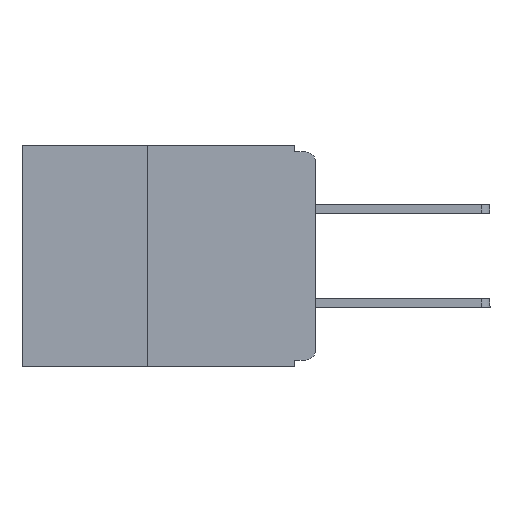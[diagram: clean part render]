
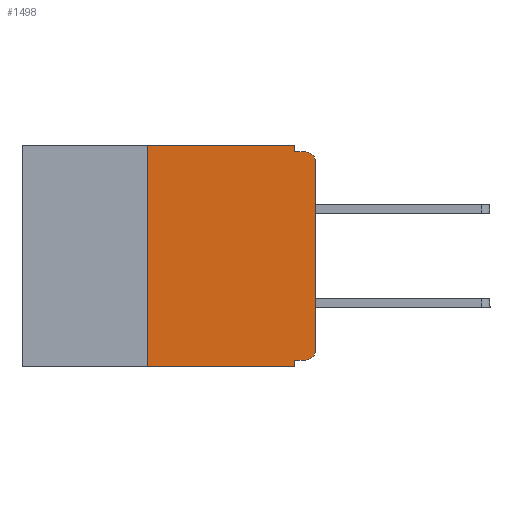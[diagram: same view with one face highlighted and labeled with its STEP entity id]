
A CAD part, left-side view. The second image highlights one B-rep face of the part: STEP entity #1498.
In plain terms, the highlighted planar face has unit normal (-1, 0, 0).
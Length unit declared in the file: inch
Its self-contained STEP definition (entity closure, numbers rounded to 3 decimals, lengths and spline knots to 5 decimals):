
#37 = EDGE_CURVE ( 'NONE', #2115, #16838, #28024, .T. ) ;
#264 = ORIENTED_EDGE ( 'NONE', *, *, #444, .F. ) ;
#444 = EDGE_CURVE ( 'NONE', #13419, #17743, #670, .T. ) ;
#670 = LINE ( 'NONE', #13961, #29350 ) ;
#885 = EDGE_CURVE ( 'NONE', #16838, #13419, #19014, .T. ) ;
#1094 = VECTOR ( 'NONE', #3043, 39.37008 ) ;
#1378 = DIRECTION ( 'NONE',  ( 0., -1., 0. ) ) ;
#1498 = ADVANCED_FACE ( 'NONE', ( #3923 ), #4084, .F. ) ;
#1636 = DIRECTION ( 'NONE',  ( -1., 0., 0. ) ) ;
#2097 = ORIENTED_EDGE ( 'NONE', *, *, #2987, .T. ) ;
#2115 = VERTEX_POINT ( 'NONE', #3869 ) ;
#2159 = CARTESIAN_POINT ( 'NONE',  ( 0., 0.437, -0.33 ) ) ;
#2605 = DIRECTION ( 'NONE',  ( 0., 0., -1. ) ) ;
#2610 = DIRECTION ( 'NONE',  ( 1., 0., 0. ) ) ;
#2978 = VERTEX_POINT ( 'NONE', #29318 ) ;
#2987 = EDGE_CURVE ( 'NONE', #21631, #26021, #19254, .T. ) ;
#3004 = VERTEX_POINT ( 'NONE', #22852 ) ;
#3043 = DIRECTION ( 'NONE',  ( 0., 0., -1. ) ) ;
#3101 = CARTESIAN_POINT ( 'NONE',  ( 0., 0.437, 0. ) ) ;
#3481 = CARTESIAN_POINT ( 'NONE',  ( 0., 0., -0.32 ) ) ;
#3617 = ORIENTED_EDGE ( 'NONE', *, *, #19073, .F. ) ;
#3869 = CARTESIAN_POINT ( 'NONE',  ( 0., 0.25, -0.33 ) ) ;
#3923 = FACE_OUTER_BOUND ( 'NONE', #14783, .T. ) ;
#3926 = VERTEX_POINT ( 'NONE', #7951 ) ;
#4084 = PLANE ( 'NONE',  #15643 ) ;
#4756 = LINE ( 'NONE', #3481, #16210 ) ;
#6631 = EDGE_CURVE ( 'NONE', #2115, #3926, #27111, .T. ) ;
#7951 = CARTESIAN_POINT ( 'NONE',  ( 0., 0.031, -0.33 ) ) ;
#8381 = AXIS2_PLACEMENT_3D ( 'NONE', #15422, #1636, #17712 ) ;
#8557 = CARTESIAN_POINT ( 'NONE',  ( 0., 0.015, -0.01 ) ) ;
#9186 = DIRECTION ( 'NONE',  ( 0., -1., 0. ) ) ;
#9751 = CARTESIAN_POINT ( 'NONE',  ( 0., 0.031, -0.01 ) ) ;
#9944 = DIRECTION ( 'NONE',  ( 0., 0., 1. ) ) ;
#10419 = CARTESIAN_POINT ( 'NONE',  ( 0., 0., -0.025 ) ) ;
#10887 = VECTOR ( 'NONE', #1378, 39.37008 ) ;
#11634 = DIRECTION ( 'NONE',  ( -1., 0., 0. ) ) ;
#11782 = CIRCLE ( 'NONE', #8381, 0.015 ) ;
#11783 = CARTESIAN_POINT ( 'NONE',  ( 0., 0.437, 0. ) ) ;
#12190 = EDGE_CURVE ( 'NONE', #2978, #25869, #11782, .T. ) ;
#12502 = DIRECTION ( 'NONE',  ( 0., -1., 0. ) ) ;
#13049 = CARTESIAN_POINT ( 'NONE',  ( 0., 0., -0.01 ) ) ;
#13100 = EDGE_CURVE ( 'NONE', #25869, #21631, #17199, .T. ) ;
#13168 = ORIENTED_EDGE ( 'NONE', *, *, #17152, .F. ) ;
#13419 = VERTEX_POINT ( 'NONE', #24625 ) ;
#13961 = CARTESIAN_POINT ( 'NONE',  ( 0., 0.031, 0. ) ) ;
#14149 = LINE ( 'NONE', #21356, #1094 ) ;
#14516 = CARTESIAN_POINT ( 'NONE',  ( 0., 0., 0. ) ) ;
#14783 = EDGE_LOOP ( 'NONE', ( #23131, #2097, #15713, #264, #16875, #15852, #19199, #3617, #13168, #15563 ) ) ;
#15422 = CARTESIAN_POINT ( 'NONE',  ( 0., 0.015, -0.305 ) ) ;
#15494 = DIRECTION ( 'NONE',  ( 0., 0., -1. ) ) ;
#15563 = ORIENTED_EDGE ( 'NONE', *, *, #12190, .T. ) ;
#15643 = AXIS2_PLACEMENT_3D ( 'NONE', #3101, #2610, #2605 ) ;
#15713 = ORIENTED_EDGE ( 'NONE', *, *, #19870, .F. ) ;
#15852 = ORIENTED_EDGE ( 'NONE', *, *, #37, .F. ) ;
#16210 = VECTOR ( 'NONE', #21755, 39.37008 ) ;
#16838 = VERTEX_POINT ( 'NONE', #20709 ) ;
#16875 = ORIENTED_EDGE ( 'NONE', *, *, #885, .F. ) ;
#17152 = EDGE_CURVE ( 'NONE', #2978, #3004, #4756, .T. ) ;
#17199 = LINE ( 'NONE', #14516, #28949 ) ;
#17712 = DIRECTION ( 'NONE',  ( 0., 0., -1. ) ) ;
#17743 = VERTEX_POINT ( 'NONE', #9751 ) ;
#19014 = LINE ( 'NONE', #11783, #25656 ) ;
#19073 = EDGE_CURVE ( 'NONE', #3004, #3926, #14149, .T. ) ;
#19199 = ORIENTED_EDGE ( 'NONE', *, *, #6631, .T. ) ;
#19254 = CIRCLE ( 'NONE', #29208, 0.015 ) ;
#19870 = EDGE_CURVE ( 'NONE', #17743, #26021, #22866, .T. ) ;
#20709 = CARTESIAN_POINT ( 'NONE',  ( 0., 0.25, 0. ) ) ;
#21199 = CARTESIAN_POINT ( 'NONE',  ( 0., 0.25, -0.33 ) ) ;
#21266 = VECTOR ( 'NONE', #9186, 39.37008 ) ;
#21356 = CARTESIAN_POINT ( 'NONE',  ( 0., 0.031, -0.33 ) ) ;
#21631 = VERTEX_POINT ( 'NONE', #10419 ) ;
#21755 = DIRECTION ( 'NONE',  ( 0., 1., 0. ) ) ;
#22222 = VECTOR ( 'NONE', #23172, 39.37008 ) ;
#22852 = CARTESIAN_POINT ( 'NONE',  ( 0., 0.031, -0.32 ) ) ;
#22866 = LINE ( 'NONE', #13049, #10887 ) ;
#23131 = ORIENTED_EDGE ( 'NONE', *, *, #13100, .T. ) ;
#23172 = DIRECTION ( 'NONE',  ( 0., 0., 1. ) ) ;
#24625 = CARTESIAN_POINT ( 'NONE',  ( 0., 0.031, 0. ) ) ;
#25116 = CARTESIAN_POINT ( 'NONE',  ( 0., 0.015, -0.025 ) ) ;
#25656 = VECTOR ( 'NONE', #12502, 39.37008 ) ;
#25869 = VERTEX_POINT ( 'NONE', #28236 ) ;
#26021 = VERTEX_POINT ( 'NONE', #8557 ) ;
#27111 = LINE ( 'NONE', #2159, #21266 ) ;
#27255 = DIRECTION ( 'NONE',  ( 0., 0., -1. ) ) ;
#28024 = LINE ( 'NONE', #21199, #22222 ) ;
#28236 = CARTESIAN_POINT ( 'NONE',  ( 0., 0., -0.305 ) ) ;
#28949 = VECTOR ( 'NONE', #9944, 39.37008 ) ;
#29208 = AXIS2_PLACEMENT_3D ( 'NONE', #25116, #11634, #27255 ) ;
#29318 = CARTESIAN_POINT ( 'NONE',  ( 0., 0.015, -0.32 ) ) ;
#29350 = VECTOR ( 'NONE', #15494, 39.37008 ) ;
